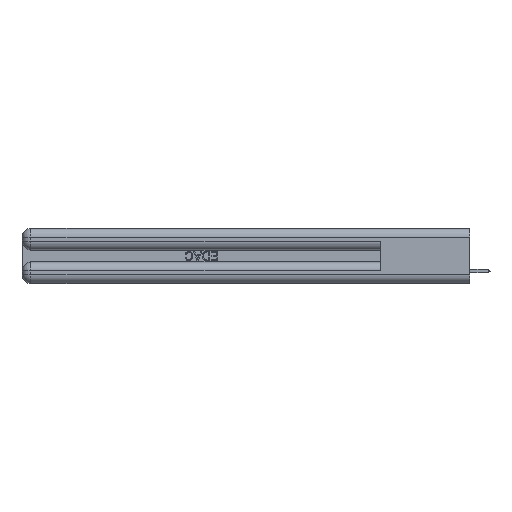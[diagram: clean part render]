
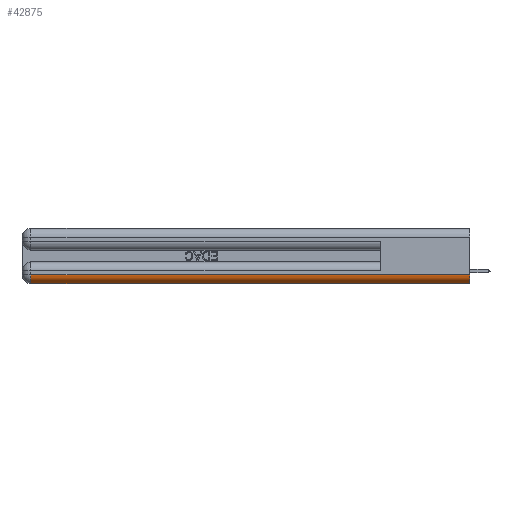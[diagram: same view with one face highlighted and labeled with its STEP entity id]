
A CAD part, left-side view. The second image highlights one B-rep face of the part: STEP entity #42875.
In plain terms, the highlighted cylindrical face has radius 1.524 mm (diameter 3.048 mm), a partial arc.
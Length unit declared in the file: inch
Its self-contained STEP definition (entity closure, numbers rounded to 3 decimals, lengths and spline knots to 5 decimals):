
#583 = ORIENTED_EDGE ( 'NONE', *, *, #12454, .F. ) ;
#629 = VERTEX_POINT ( 'NONE', #3097 ) ;
#731 = VERTEX_POINT ( 'NONE', #47127 ) ;
#3097 = CARTESIAN_POINT ( 'NONE',  ( 0., 0., 0.06 ) ) ;
#4168 = CIRCLE ( 'NONE', #47642, 0.06 ) ;
#4600 = AXIS2_PLACEMENT_3D ( 'NONE', #45518, #34356, #12277 ) ;
#5744 = VERTEX_POINT ( 'NONE', #35491 ) ;
#6764 = CARTESIAN_POINT ( 'NONE',  ( 0.06, 0., 0.06 ) ) ;
#8797 = LINE ( 'NONE', #17465, #41693 ) ;
#10529 = DIRECTION ( 'NONE',  ( 0., 0., 1. ) ) ;
#11447 = CARTESIAN_POINT ( 'NONE',  ( 0.06, 0., 0.06 ) ) ;
#11686 = VECTOR ( 'NONE', #12485, 39.37008 ) ;
#12277 = DIRECTION ( 'NONE',  ( 0., 0., 1. ) ) ;
#12328 = CARTESIAN_POINT ( 'NONE',  ( 0.06, 3., 0. ) ) ;
#12454 = EDGE_CURVE ( 'NONE', #39313, #629, #8797, .T. ) ;
#12485 = DIRECTION ( 'NONE',  ( 0., 1., 0. ) ) ;
#14360 = ORIENTED_EDGE ( 'NONE', *, *, #27409, .F. ) ;
#15479 = DIRECTION ( 'NONE',  ( 0., 0., 1. ) ) ;
#15879 = CIRCLE ( 'NONE', #4600, 0.06 ) ;
#17465 = CARTESIAN_POINT ( 'NONE',  ( 0., 0., 0.06 ) ) ;
#18247 = DIRECTION ( 'NONE',  ( 0., 1., 0. ) ) ;
#18397 = ORIENTED_EDGE ( 'NONE', *, *, #21636, .F. ) ;
#19320 = EDGE_LOOP ( 'NONE', ( #24123, #583, #18397, #14360 ) ) ;
#21494 = DIRECTION ( 'NONE',  ( 0., -1., 0. ) ) ;
#21636 = EDGE_CURVE ( 'NONE', #731, #39313, #15879, .T. ) ;
#24123 = ORIENTED_EDGE ( 'NONE', *, *, #30141, .F. ) ;
#26138 = LINE ( 'NONE', #12328, #11686 ) ;
#26293 = AXIS2_PLACEMENT_3D ( 'NONE', #6764, #18247, #10529 ) ;
#27409 = EDGE_CURVE ( 'NONE', #5744, #731, #26138, .T. ) ;
#29988 = DIRECTION ( 'NONE',  ( 0., -1., 0. ) ) ;
#30141 = EDGE_CURVE ( 'NONE', #629, #5744, #4168, .T. ) ;
#34356 = DIRECTION ( 'NONE',  ( 0., 1., 0. ) ) ;
#35491 = CARTESIAN_POINT ( 'NONE',  ( 0.06, 0., 0. ) ) ;
#39313 = VERTEX_POINT ( 'NONE', #47438 ) ;
#41546 = CYLINDRICAL_SURFACE ( 'NONE', #26293, 0.06 ) ;
#41693 = VECTOR ( 'NONE', #21494, 39.37008 ) ;
#42206 = FACE_OUTER_BOUND ( 'NONE', #19320, .T. ) ;
#42875 = ADVANCED_FACE ( 'NONE', ( #42206 ), #41546, .T. ) ;
#45518 = CARTESIAN_POINT ( 'NONE',  ( 0.06, 2.94, 0.06 ) ) ;
#47127 = CARTESIAN_POINT ( 'NONE',  ( 0.06, 2.94, 0. ) ) ;
#47438 = CARTESIAN_POINT ( 'NONE',  ( 0., 2.94, 0.06 ) ) ;
#47642 = AXIS2_PLACEMENT_3D ( 'NONE', #11447, #29988, #15479 ) ;
